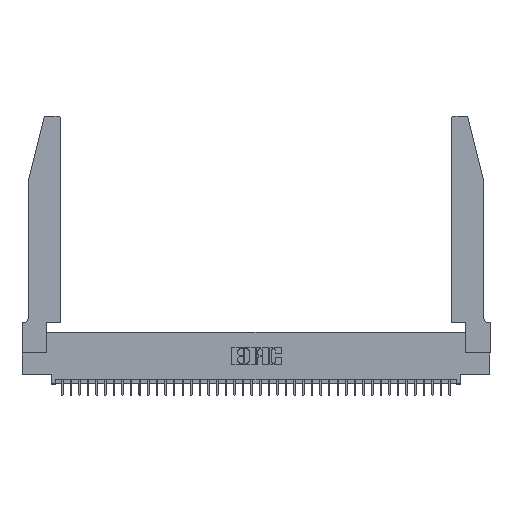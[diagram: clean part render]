
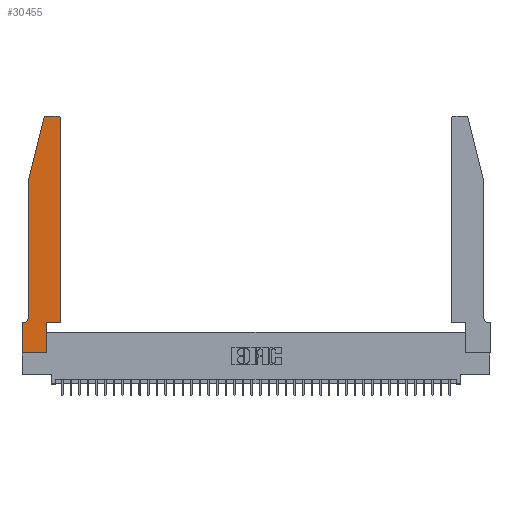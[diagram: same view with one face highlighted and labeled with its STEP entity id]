
A CAD part, top view. The second image highlights one B-rep face of the part: STEP entity #30455.
In plain terms, the highlighted planar face has unit normal (0, 0, 1).
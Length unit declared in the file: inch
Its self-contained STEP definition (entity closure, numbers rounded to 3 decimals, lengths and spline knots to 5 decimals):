
#260 = ORIENTED_EDGE ( 'NONE', *, *, #36245, .T. ) ;
#1534 = DIRECTION ( 'NONE',  ( 0., 0., -1. ) ) ;
#2007 = VECTOR ( 'NONE', #7783, 39.37008 ) ;
#3739 = CARTESIAN_POINT ( 'NONE',  ( 0.284, 2.75, 0.37 ) ) ;
#4061 = CARTESIAN_POINT ( 'NONE',  ( 0.25487, 2.72718, 0.37 ) ) ;
#4096 = LINE ( 'NONE', #7390, #2007 ) ;
#4852 = EDGE_CURVE ( 'NONE', #22430, #23033, #29145, .T. ) ;
#5277 = VECTOR ( 'NONE', #18756, 39.37008 ) ;
#5394 = VERTEX_POINT ( 'NONE', #21578 ) ;
#5401 = ORIENTED_EDGE ( 'NONE', *, *, #15829, .T. ) ;
#5876 = VERTEX_POINT ( 'NONE', #4061 ) ;
#6241 = CARTESIAN_POINT ( 'NONE',  ( 0.2605, 2.75, 0.37 ) ) ;
#6335 = FACE_OUTER_BOUND ( 'NONE', #31486, .T. ) ;
#7390 = CARTESIAN_POINT ( 'NONE',  ( 0.0755, 2., 0.37 ) ) ;
#7782 = EDGE_CURVE ( 'NONE', #27403, #5394, #17536, .T. ) ;
#7783 = DIRECTION ( 'NONE',  ( -0.239, -0.971, 0. ) ) ;
#8414 = EDGE_CURVE ( 'NONE', #25837, #22430, #11790, .T. ) ;
#8968 = EDGE_CURVE ( 'NONE', #5394, #25837, #37149, .T. ) ;
#9006 = DIRECTION ( 'NONE',  ( 0., 0., 1. ) ) ;
#9024 = DIRECTION ( 'NONE',  ( 1., 0., 0. ) ) ;
#9337 = AXIS2_PLACEMENT_3D ( 'NONE', #21046, #1534, #14272 ) ;
#10305 = VECTOR ( 'NONE', #35070, 39.37008 ) ;
#11568 = DIRECTION ( 'NONE',  ( 1., 0., 0. ) ) ;
#11790 = LINE ( 'NONE', #31307, #15538 ) ;
#11879 = DIRECTION ( 'NONE',  ( 1., 0., 0. ) ) ;
#12171 = ORIENTED_EDGE ( 'NONE', *, *, #18923, .T. ) ;
#12659 = DIRECTION ( 'NONE',  ( 0., 0., 1. ) ) ;
#13333 = CARTESIAN_POINT ( 'NONE',  ( 0.4205, 2.75, 0.37 ) ) ;
#13540 = CARTESIAN_POINT ( 'NONE',  ( 0.0755, 0.42, 0.37 ) ) ;
#13801 = EDGE_CURVE ( 'NONE', #15178, #22084, #20561, .T. ) ;
#14010 = CARTESIAN_POINT ( 'NONE',  ( 0.0055, 0.35, 0.37 ) ) ;
#14065 = CARTESIAN_POINT ( 'NONE',  ( 0.2865, 0.35, 0.37 ) ) ;
#14272 = DIRECTION ( 'NONE',  ( -1., 0., 0. ) ) ;
#14689 = DIRECTION ( 'NONE',  ( 0., 1., 0. ) ) ;
#14876 = VECTOR ( 'NONE', #36006, 39.37008 ) ;
#15168 = CARTESIAN_POINT ( 'NONE',  ( 0., 0.35, 0.37 ) ) ;
#15178 = VERTEX_POINT ( 'NONE', #14010 ) ;
#15538 = VECTOR ( 'NONE', #14689, 39.37008 ) ;
#15829 = EDGE_CURVE ( 'NONE', #17308, #21832, #22553, .T. ) ;
#17119 = ORIENTED_EDGE ( 'NONE', *, *, #4852, .T. ) ;
#17308 = VERTEX_POINT ( 'NONE', #23418 ) ;
#17536 = LINE ( 'NONE', #14065, #14876 ) ;
#17903 = EDGE_CURVE ( 'NONE', #23033, #32498, #33821, .T. ) ;
#18325 = CARTESIAN_POINT ( 'NONE',  ( 0.4205, 2.72, 0.37 ) ) ;
#18756 = DIRECTION ( 'NONE',  ( -1., 0., 0. ) ) ;
#18923 = EDGE_CURVE ( 'NONE', #21677, #27403, #22555, .T. ) ;
#20281 = DIRECTION ( 'NONE',  ( 0., -1., 0. ) ) ;
#20561 = LINE ( 'NONE', #29620, #27780 ) ;
#21046 = CARTESIAN_POINT ( 'NONE',  ( 0.0055, 0.42, 0.37 ) ) ;
#21578 = CARTESIAN_POINT ( 'NONE',  ( 0.2865, 0.35, 0.37 ) ) ;
#21677 = VERTEX_POINT ( 'NONE', #31630 ) ;
#21738 = EDGE_CURVE ( 'NONE', #5876, #17308, #4096, .T. ) ;
#21783 = ORIENTED_EDGE ( 'NONE', *, *, #13801, .T. ) ;
#21832 = VERTEX_POINT ( 'NONE', #13540 ) ;
#22084 = VERTEX_POINT ( 'NONE', #15168 ) ;
#22430 = VERTEX_POINT ( 'NONE', #24523 ) ;
#22553 = LINE ( 'NONE', #31602, #10305 ) ;
#22555 = LINE ( 'NONE', #40428, #30195 ) ;
#23033 = VERTEX_POINT ( 'NONE', #13333 ) ;
#23210 = AXIS2_PLACEMENT_3D ( 'NONE', #18325, #30878, #37222 ) ;
#23416 = ORIENTED_EDGE ( 'NONE', *, *, #21738, .T. ) ;
#23418 = CARTESIAN_POINT ( 'NONE',  ( 0.0755, 2., 0.37 ) ) ;
#24108 = EDGE_CURVE ( 'NONE', #21832, #15178, #25085, .T. ) ;
#24523 = CARTESIAN_POINT ( 'NONE',  ( 0.4505, 2.72, 0.37 ) ) ;
#24987 = CIRCLE ( 'NONE', #27635, 0.03 ) ;
#25085 = CIRCLE ( 'NONE', #9337, 0.07 ) ;
#25228 = PLANE ( 'NONE',  #29790 ) ;
#25837 = VERTEX_POINT ( 'NONE', #30976 ) ;
#27403 = VERTEX_POINT ( 'NONE', #36247 ) ;
#27522 = ORIENTED_EDGE ( 'NONE', *, *, #24108, .T. ) ;
#27635 = AXIS2_PLACEMENT_3D ( 'NONE', #30968, #12659, #34622 ) ;
#27780 = VECTOR ( 'NONE', #33090, 39.37008 ) ;
#29145 = CIRCLE ( 'NONE', #23210, 0.03 ) ;
#29360 = VECTOR ( 'NONE', #9024, 39.37008 ) ;
#29620 = CARTESIAN_POINT ( 'NONE',  ( 0.0755, 0.35, 0.37 ) ) ;
#29630 = ORIENTED_EDGE ( 'NONE', *, *, #17903, .T. ) ;
#29750 = LINE ( 'NONE', #33007, #39411 ) ;
#29790 = AXIS2_PLACEMENT_3D ( 'NONE', #34045, #9006, #11879 ) ;
#30195 = VECTOR ( 'NONE', #11568, 39.37008 ) ;
#30455 = ADVANCED_FACE ( 'NONE', ( #6335 ), #25228, .T. ) ;
#30878 = DIRECTION ( 'NONE',  ( 0., 0., 1. ) ) ;
#30968 = CARTESIAN_POINT ( 'NONE',  ( 0.284, 2.72, 0.37 ) ) ;
#30976 = CARTESIAN_POINT ( 'NONE',  ( 0.4505, 0.35, 0.37 ) ) ;
#31005 = CARTESIAN_POINT ( 'NONE',  ( 0.4505, 0.35, 0.37 ) ) ;
#31307 = CARTESIAN_POINT ( 'NONE',  ( 0.4505, 0.35, 0.37 ) ) ;
#31486 = EDGE_LOOP ( 'NONE', ( #29630, #32839, #23416, #5401, #27522, #21783, #260, #12171, #38637, #34247, #39534, #17119 ) ) ;
#31602 = CARTESIAN_POINT ( 'NONE',  ( 0.0755, 2., 0.37 ) ) ;
#31630 = CARTESIAN_POINT ( 'NONE',  ( 0., 0., 0.37 ) ) ;
#32498 = VERTEX_POINT ( 'NONE', #3739 ) ;
#32839 = ORIENTED_EDGE ( 'NONE', *, *, #37905, .T. ) ;
#33007 = CARTESIAN_POINT ( 'NONE',  ( 0., 0., 0.37 ) ) ;
#33090 = DIRECTION ( 'NONE',  ( -1., 0., 0. ) ) ;
#33821 = LINE ( 'NONE', #6241, #5277 ) ;
#34045 = CARTESIAN_POINT ( 'NONE',  ( 0., 0.35, 0.37 ) ) ;
#34247 = ORIENTED_EDGE ( 'NONE', *, *, #8968, .T. ) ;
#34622 = DIRECTION ( 'NONE',  ( 1., 0., 0. ) ) ;
#35070 = DIRECTION ( 'NONE',  ( 0., -1., 0. ) ) ;
#36006 = DIRECTION ( 'NONE',  ( 0., 1., 0. ) ) ;
#36245 = EDGE_CURVE ( 'NONE', #22084, #21677, #29750, .T. ) ;
#36247 = CARTESIAN_POINT ( 'NONE',  ( 0.2865, 0., 0.37 ) ) ;
#37149 = LINE ( 'NONE', #31005, #29360 ) ;
#37222 = DIRECTION ( 'NONE',  ( 1., 0., 0. ) ) ;
#37905 = EDGE_CURVE ( 'NONE', #32498, #5876, #24987, .T. ) ;
#38637 = ORIENTED_EDGE ( 'NONE', *, *, #7782, .T. ) ;
#39411 = VECTOR ( 'NONE', #20281, 39.37008 ) ;
#39534 = ORIENTED_EDGE ( 'NONE', *, *, #8414, .T. ) ;
#40428 = CARTESIAN_POINT ( 'NONE',  ( 0., 0., 0.37 ) ) ;
